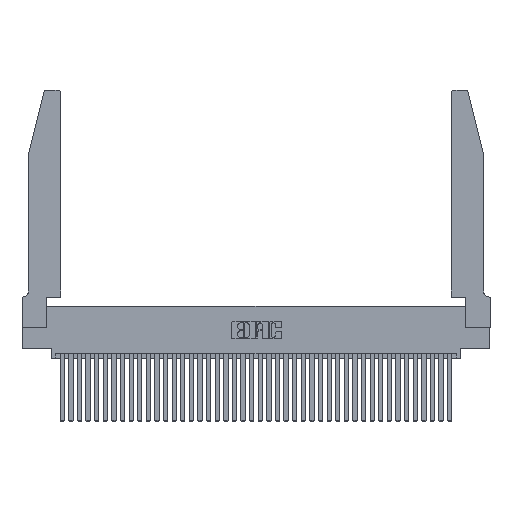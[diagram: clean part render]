
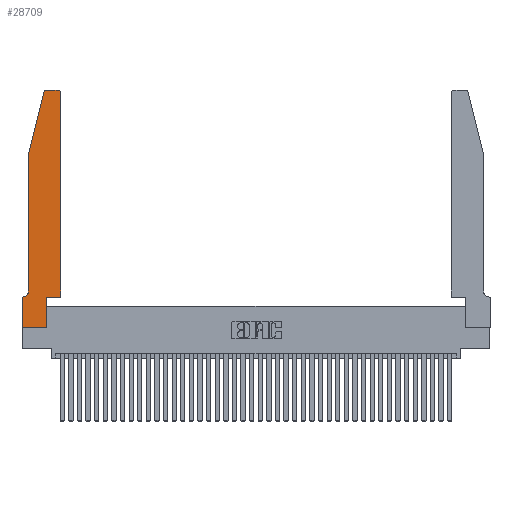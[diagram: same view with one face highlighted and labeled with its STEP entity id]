
A CAD part, top view. The second image highlights one B-rep face of the part: STEP entity #28709.
In plain terms, the highlighted planar face has unit normal (0, 0, 1).
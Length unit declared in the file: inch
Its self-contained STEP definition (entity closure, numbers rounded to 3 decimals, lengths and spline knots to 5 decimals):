
#242 = VECTOR ( 'NONE', #13019, 39.37008 ) ;
#1186 = CARTESIAN_POINT ( 'NONE',  ( 0.4505, 0.35, 0.37 ) ) ;
#1519 = CARTESIAN_POINT ( 'NONE',  ( 0.284, 2.75, 0.37 ) ) ;
#1565 = DIRECTION ( 'NONE',  ( 1., 0., 0. ) ) ;
#1772 = EDGE_CURVE ( 'NONE', #8505, #31351, #17234, .T. ) ;
#2303 = VERTEX_POINT ( 'NONE', #17731 ) ;
#3005 = DIRECTION ( 'NONE',  ( 1., 0., 0. ) ) ;
#3976 = DIRECTION ( 'NONE',  ( 1., 0., 0. ) ) ;
#4135 = VECTOR ( 'NONE', #35116, 39.37008 ) ;
#5156 = ORIENTED_EDGE ( 'NONE', *, *, #1772, .T. ) ;
#5348 = EDGE_CURVE ( 'NONE', #33299, #11132, #38075, .T. ) ;
#5462 = EDGE_CURVE ( 'NONE', #36352, #21507, #37619, .T. ) ;
#5926 = DIRECTION ( 'NONE',  ( 1., 0., 0. ) ) ;
#6007 = VERTEX_POINT ( 'NONE', #24094 ) ;
#6030 = AXIS2_PLACEMENT_3D ( 'NONE', #34209, #34476, #18896 ) ;
#6517 = LINE ( 'NONE', #37959, #30872 ) ;
#6562 = EDGE_CURVE ( 'NONE', #13486, #13900, #36544, .T. ) ;
#6619 = ORIENTED_EDGE ( 'NONE', *, *, #11039, .T. ) ;
#7077 = DIRECTION ( 'NONE',  ( 0., 0., 1. ) ) ;
#7192 = CIRCLE ( 'NONE', #31603, 0.03 ) ;
#7527 = CARTESIAN_POINT ( 'NONE',  ( 0., 0.35, 0.37 ) ) ;
#8505 = VERTEX_POINT ( 'NONE', #30476 ) ;
#8794 = CARTESIAN_POINT ( 'NONE',  ( 0.2605, 2.75, 0.37 ) ) ;
#8980 = VECTOR ( 'NONE', #10982, 39.37008 ) ;
#9445 = LINE ( 'NONE', #29467, #8980 ) ;
#9752 = EDGE_CURVE ( 'NONE', #13900, #2303, #33823, .T. ) ;
#10011 = CARTESIAN_POINT ( 'NONE',  ( 0.0055, 0.35, 0.37 ) ) ;
#10244 = ORIENTED_EDGE ( 'NONE', *, *, #21546, .T. ) ;
#10982 = DIRECTION ( 'NONE',  ( 0., -1., 0. ) ) ;
#11039 = EDGE_CURVE ( 'NONE', #11132, #6007, #36155, .T. ) ;
#11132 = VERTEX_POINT ( 'NONE', #1519 ) ;
#11180 = ORIENTED_EDGE ( 'NONE', *, *, #5348, .T. ) ;
#12629 = CARTESIAN_POINT ( 'NONE',  ( 0., 0.35, 0.37 ) ) ;
#12792 = VECTOR ( 'NONE', #5926, 39.37008 ) ;
#13019 = DIRECTION ( 'NONE',  ( 0., 1., 0. ) ) ;
#13355 = CARTESIAN_POINT ( 'NONE',  ( 0.0755, 2., 0.37 ) ) ;
#13486 = VERTEX_POINT ( 'NONE', #14493 ) ;
#13797 = ORIENTED_EDGE ( 'NONE', *, *, #24008, .T. ) ;
#13900 = VERTEX_POINT ( 'NONE', #39106 ) ;
#14485 = ORIENTED_EDGE ( 'NONE', *, *, #35672, .T. ) ;
#14493 = CARTESIAN_POINT ( 'NONE',  ( 0.2865, 0.35, 0.37 ) ) ;
#15231 = DIRECTION ( 'NONE',  ( -1., 0., 0. ) ) ;
#15644 = CARTESIAN_POINT ( 'NONE',  ( 0.4505, 0.35, 0.37 ) ) ;
#15970 = DIRECTION ( 'NONE',  ( 0., 1., 0. ) ) ;
#16256 = CARTESIAN_POINT ( 'NONE',  ( 0.284, 2.72, 0.37 ) ) ;
#17234 = LINE ( 'NONE', #13355, #29282 ) ;
#17731 = CARTESIAN_POINT ( 'NONE',  ( 0.4505, 2.72, 0.37 ) ) ;
#18134 = DIRECTION ( 'NONE',  ( -1., 0., 0. ) ) ;
#18896 = DIRECTION ( 'NONE',  ( -1., 0., 0. ) ) ;
#19051 = DIRECTION ( 'NONE',  ( 1., 0., 0. ) ) ;
#20037 = VECTOR ( 'NONE', #19051, 39.37008 ) ;
#20184 = ORIENTED_EDGE ( 'NONE', *, *, #25960, .T. ) ;
#20242 = PLANE ( 'NONE',  #38727 ) ;
#21507 = VERTEX_POINT ( 'NONE', #32740 ) ;
#21546 = EDGE_CURVE ( 'NONE', #33442, #36352, #9445, .T. ) ;
#21760 = CARTESIAN_POINT ( 'NONE',  ( 0.4205, 2.72, 0.37 ) ) ;
#23076 = EDGE_CURVE ( 'NONE', #31351, #27976, #40031, .T. ) ;
#24008 = EDGE_CURVE ( 'NONE', #27976, #33442, #32210, .T. ) ;
#24045 = LINE ( 'NONE', #29243, #4135 ) ;
#24094 = CARTESIAN_POINT ( 'NONE',  ( 0.25487, 2.72718, 0.37 ) ) ;
#25960 = EDGE_CURVE ( 'NONE', #2303, #33299, #7192, .T. ) ;
#26806 = CARTESIAN_POINT ( 'NONE',  ( 0.0755, 0.42, 0.37 ) ) ;
#26991 = ORIENTED_EDGE ( 'NONE', *, *, #23076, .T. ) ;
#27976 = VERTEX_POINT ( 'NONE', #10011 ) ;
#28709 = ADVANCED_FACE ( 'NONE', ( #35070 ), #20242, .T. ) ;
#29226 = ORIENTED_EDGE ( 'NONE', *, *, #6562, .T. ) ;
#29243 = CARTESIAN_POINT ( 'NONE',  ( 0.0755, 2., 0.37 ) ) ;
#29282 = VECTOR ( 'NONE', #39557, 39.37008 ) ;
#29467 = CARTESIAN_POINT ( 'NONE',  ( 0., 0., 0.37 ) ) ;
#29654 = ORIENTED_EDGE ( 'NONE', *, *, #5462, .T. ) ;
#29683 = AXIS2_PLACEMENT_3D ( 'NONE', #16256, #7077, #3976 ) ;
#29838 = CARTESIAN_POINT ( 'NONE',  ( 0., 0., 0.37 ) ) ;
#30303 = VECTOR ( 'NONE', #15231, 39.37008 ) ;
#30476 = CARTESIAN_POINT ( 'NONE',  ( 0.0755, 2., 0.37 ) ) ;
#30872 = VECTOR ( 'NONE', #15970, 39.37008 ) ;
#31351 = VERTEX_POINT ( 'NONE', #26806 ) ;
#31603 = AXIS2_PLACEMENT_3D ( 'NONE', #21760, #37261, #3005 ) ;
#32210 = LINE ( 'NONE', #39715, #36148 ) ;
#32740 = CARTESIAN_POINT ( 'NONE',  ( 0.2865, 0., 0.37 ) ) ;
#32763 = EDGE_CURVE ( 'NONE', #21507, #13486, #6517, .T. ) ;
#33299 = VERTEX_POINT ( 'NONE', #39857 ) ;
#33442 = VERTEX_POINT ( 'NONE', #12629 ) ;
#33823 = LINE ( 'NONE', #1186, #242 ) ;
#34209 = CARTESIAN_POINT ( 'NONE',  ( 0.0055, 0.42, 0.37 ) ) ;
#34222 = EDGE_LOOP ( 'NONE', ( #11180, #6619, #14485, #5156, #26991, #13797, #10244, #29654, #36618, #29226, #35298, #20184 ) ) ;
#34476 = DIRECTION ( 'NONE',  ( 0., 0., -1. ) ) ;
#35070 = FACE_OUTER_BOUND ( 'NONE', #34222, .T. ) ;
#35116 = DIRECTION ( 'NONE',  ( -0.239, -0.971, 0. ) ) ;
#35298 = ORIENTED_EDGE ( 'NONE', *, *, #9752, .T. ) ;
#35566 = DIRECTION ( 'NONE',  ( 0., 0., 1. ) ) ;
#35672 = EDGE_CURVE ( 'NONE', #6007, #8505, #24045, .T. ) ;
#36148 = VECTOR ( 'NONE', #18134, 39.37008 ) ;
#36155 = CIRCLE ( 'NONE', #29683, 0.03 ) ;
#36352 = VERTEX_POINT ( 'NONE', #38055 ) ;
#36544 = LINE ( 'NONE', #15644, #20037 ) ;
#36618 = ORIENTED_EDGE ( 'NONE', *, *, #32763, .T. ) ;
#37261 = DIRECTION ( 'NONE',  ( 0., 0., 1. ) ) ;
#37619 = LINE ( 'NONE', #29838, #12792 ) ;
#37959 = CARTESIAN_POINT ( 'NONE',  ( 0.2865, 0.35, 0.37 ) ) ;
#38055 = CARTESIAN_POINT ( 'NONE',  ( 0., 0., 0.37 ) ) ;
#38075 = LINE ( 'NONE', #8794, #30303 ) ;
#38727 = AXIS2_PLACEMENT_3D ( 'NONE', #7527, #35566, #1565 ) ;
#39106 = CARTESIAN_POINT ( 'NONE',  ( 0.4505, 0.35, 0.37 ) ) ;
#39557 = DIRECTION ( 'NONE',  ( 0., -1., 0. ) ) ;
#39715 = CARTESIAN_POINT ( 'NONE',  ( 0.0755, 0.35, 0.37 ) ) ;
#39857 = CARTESIAN_POINT ( 'NONE',  ( 0.4205, 2.75, 0.37 ) ) ;
#40031 = CIRCLE ( 'NONE', #6030, 0.07 ) ;
